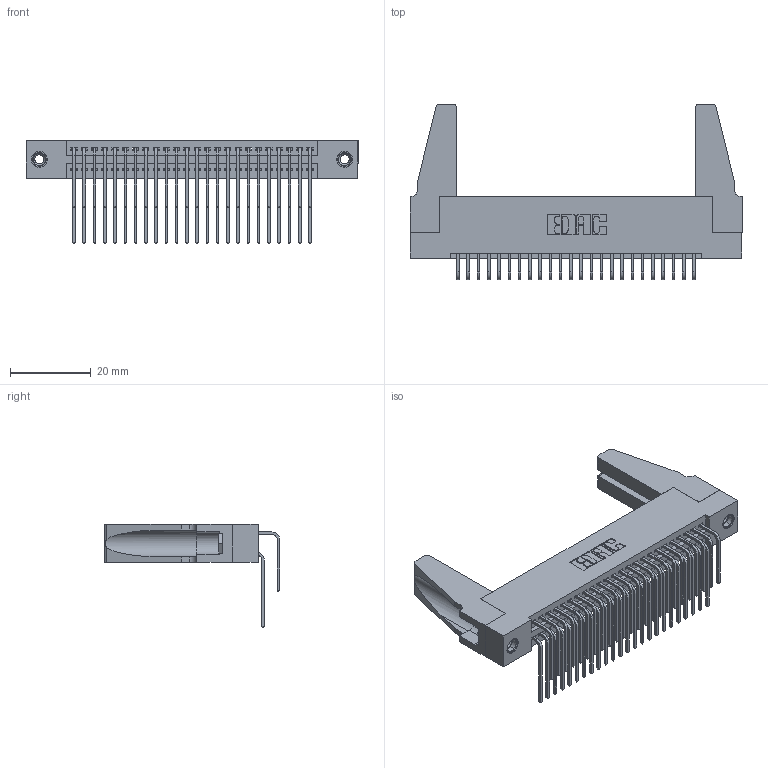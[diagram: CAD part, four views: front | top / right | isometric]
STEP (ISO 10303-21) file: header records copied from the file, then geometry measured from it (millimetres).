
FILE_DESCRIPTION (( 'STEP AP203' ), '1' );
FILE_NAME ('345-048-559-288.STEP', '2019-10-29T06:02:09', ( '' ), ( '' ), 'SwSTEP 2.0', 'SolidWorks 2016', '' );
FILE_SCHEMA (( 'CONFIG_CONTROL_DESIGN' ));
Length unit declared in the file: inch
Products named in the file (6): 345-250-001_345-250-001-102; 345-048-559-288; 345 Part_Flush Mounting Lugs - 0.156 Dia-TH; 345-292-001_558 559 Tail - 1; 345-220-078_345-220-088; 345-292-001_559 Tail - 2
Assembly tree (53 placements, depth 2):
  345-048-559-288
    345 Part_Flush Mounting Lugs - 0.156 Dia-TH
    345-292-001_558 559 Tail - 1  x24
    345-292-001_559 Tail - 2  x24
    345-250-001_345-250-001-102  x2
    345-220-078_345-220-088  x2
Bounding box: 82.19 x 43.42 x 25.53 mm (x, y, z)
Volume: 11346.7 mm3; surface area: 16040.3 mm2
Topology: 53 solids, 53 shells, 2746 faces, 8095 edges, 5322 vertices
Faces by surface type: plane 1832, cylinder 898, cone 12, torus 4
Entity records: 25054 total; most frequent: CARTESIAN_POINT 4257, ORIENTED_EDGE 4100, DIRECTION 3754, EDGE_CURVE 2050, LINE 1740, VECTOR 1740, VERTEX_POINT 1358, AXIS2_PLACEMENT_3D 1007
